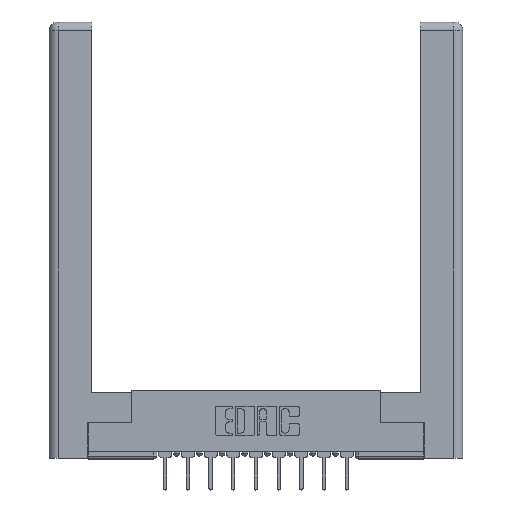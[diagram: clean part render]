
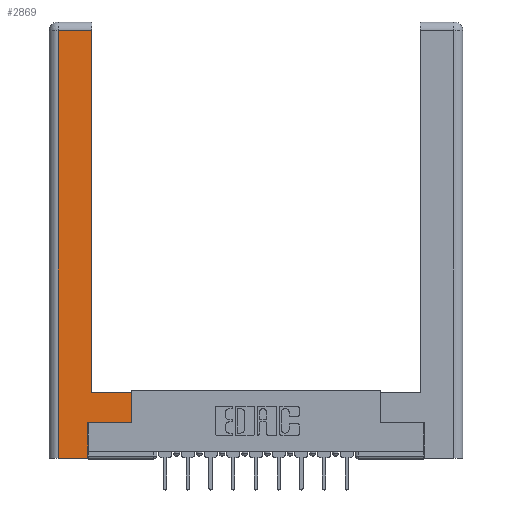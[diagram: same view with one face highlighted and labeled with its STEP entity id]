
A CAD part, top view. The second image highlights one B-rep face of the part: STEP entity #2869.
In plain terms, the highlighted planar face has unit normal (0, 0, 1).
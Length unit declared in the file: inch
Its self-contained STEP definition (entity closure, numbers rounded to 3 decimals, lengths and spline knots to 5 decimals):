
#224 = DIRECTION ( 'NONE',  ( 0., -1., 0. ) ) ;
#247 = ORIENTED_EDGE ( 'NONE', *, *, #12027, .T. ) ;
#271 = ORIENTED_EDGE ( 'NONE', *, *, #11911, .T. ) ;
#418 = LINE ( 'NONE', #1720, #6188 ) ;
#782 = CARTESIAN_POINT ( 'NONE',  ( 0.265, 0., 0. ) ) ;
#951 = VERTEX_POINT ( 'NONE', #11883 ) ;
#1154 = VERTEX_POINT ( 'NONE', #10119 ) ;
#1720 = CARTESIAN_POINT ( 'NONE',  ( 0.565, 0.45, 0. ) ) ;
#2081 = ORIENTED_EDGE ( 'NONE', *, *, #4164, .T. ) ;
#2122 = CARTESIAN_POINT ( 'NONE',  ( 0.565, 0.245, 0. ) ) ;
#2341 = LINE ( 'NONE', #7872, #5028 ) ;
#2370 = DIRECTION ( 'NONE',  ( 0., 0., -1. ) ) ;
#2428 = EDGE_LOOP ( 'NONE', ( #247, #7241, #2081, #8411, #6147, #271, #4485, #8928 ) ) ;
#2704 = VECTOR ( 'NONE', #11024, 39.37008 ) ;
#2837 = EDGE_CURVE ( 'NONE', #10962, #11419, #12298, .T. ) ;
#2869 = ADVANCED_FACE ( 'NONE', ( #4625 ), #12372, .F. ) ;
#3006 = CARTESIAN_POINT ( 'NONE',  ( 0.265, 0.245, 0. ) ) ;
#3291 = VERTEX_POINT ( 'NONE', #3360 ) ;
#3360 = CARTESIAN_POINT ( 'NONE',  ( 0.295, 2.94, 0. ) ) ;
#3362 = VECTOR ( 'NONE', #9673, 39.37008 ) ;
#3974 = VERTEX_POINT ( 'NONE', #11956 ) ;
#4154 = LINE ( 'NONE', #2122, #2704 ) ;
#4164 = EDGE_CURVE ( 'NONE', #951, #3974, #13778, .T. ) ;
#4485 = ORIENTED_EDGE ( 'NONE', *, *, #9574, .T. ) ;
#4625 = FACE_OUTER_BOUND ( 'NONE', #2428, .T. ) ;
#4885 = VECTOR ( 'NONE', #6746, 39.37008 ) ;
#5028 = VECTOR ( 'NONE', #7939, 39.37008 ) ;
#5196 = CARTESIAN_POINT ( 'NONE',  ( 0.295, 0.45, 0. ) ) ;
#6147 = ORIENTED_EDGE ( 'NONE', *, *, #2837, .T. ) ;
#6155 = LINE ( 'NONE', #5196, #3362 ) ;
#6173 = VECTOR ( 'NONE', #13279, 39.37008 ) ;
#6188 = VECTOR ( 'NONE', #7032, 39.37008 ) ;
#6381 = CARTESIAN_POINT ( 'NONE',  ( 0.265, 0., 0. ) ) ;
#6626 = CARTESIAN_POINT ( 'NONE',  ( 0.565, 0.245, 0. ) ) ;
#6746 = DIRECTION ( 'NONE',  ( 0., 1., 0. ) ) ;
#6811 = DIRECTION ( 'NONE',  ( -1., 0., 0. ) ) ;
#6831 = VERTEX_POINT ( 'NONE', #12167 ) ;
#7032 = DIRECTION ( 'NONE',  ( 0., 1., 0. ) ) ;
#7063 = EDGE_CURVE ( 'NONE', #3974, #10962, #10774, .T. ) ;
#7078 = EDGE_CURVE ( 'NONE', #6831, #1154, #6155, .T. ) ;
#7241 = ORIENTED_EDGE ( 'NONE', *, *, #9359, .T. ) ;
#7872 = CARTESIAN_POINT ( 'NONE',  ( 0.295, 3., 0. ) ) ;
#7939 = DIRECTION ( 'NONE',  ( 0., 1., 0. ) ) ;
#8411 = ORIENTED_EDGE ( 'NONE', *, *, #7063, .T. ) ;
#8859 = VERTEX_POINT ( 'NONE', #6626 ) ;
#8928 = ORIENTED_EDGE ( 'NONE', *, *, #7078, .T. ) ;
#9315 = CARTESIAN_POINT ( 'NONE',  ( 0.0615, 0., 0. ) ) ;
#9359 = EDGE_CURVE ( 'NONE', #3291, #951, #14280, .T. ) ;
#9574 = EDGE_CURVE ( 'NONE', #8859, #6831, #418, .T. ) ;
#9663 = VECTOR ( 'NONE', #11652, 39.37008 ) ;
#9673 = DIRECTION ( 'NONE',  ( -1., 0., 0. ) ) ;
#10106 = CARTESIAN_POINT ( 'NONE',  ( 0., 0., 0. ) ) ;
#10119 = CARTESIAN_POINT ( 'NONE',  ( 0.295, 0.45, 0. ) ) ;
#10306 = VECTOR ( 'NONE', #224, 39.37008 ) ;
#10774 = LINE ( 'NONE', #782, #9663 ) ;
#10962 = VERTEX_POINT ( 'NONE', #6381 ) ;
#11024 = DIRECTION ( 'NONE',  ( 1., 0., 0. ) ) ;
#11419 = VERTEX_POINT ( 'NONE', #3006 ) ;
#11427 = CARTESIAN_POINT ( 'NONE',  ( 0.265, 0.245, 0. ) ) ;
#11652 = DIRECTION ( 'NONE',  ( 1., 0., 0. ) ) ;
#11883 = CARTESIAN_POINT ( 'NONE',  ( 0.0615, 2.94, 0. ) ) ;
#11911 = EDGE_CURVE ( 'NONE', #11419, #8859, #4154, .T. ) ;
#11956 = CARTESIAN_POINT ( 'NONE',  ( 0.0615, 0., 0. ) ) ;
#12027 = EDGE_CURVE ( 'NONE', #1154, #3291, #2341, .T. ) ;
#12167 = CARTESIAN_POINT ( 'NONE',  ( 0.565, 0.45, 0. ) ) ;
#12298 = LINE ( 'NONE', #11427, #4885 ) ;
#12372 = PLANE ( 'NONE',  #12378 ) ;
#12378 = AXIS2_PLACEMENT_3D ( 'NONE', #10106, #2370, #6811 ) ;
#13201 = CARTESIAN_POINT ( 'NONE',  ( 0.0615, 2.94, 0. ) ) ;
#13279 = DIRECTION ( 'NONE',  ( -1., 0., 0. ) ) ;
#13778 = LINE ( 'NONE', #9315, #10306 ) ;
#14280 = LINE ( 'NONE', #13201, #6173 ) ;
